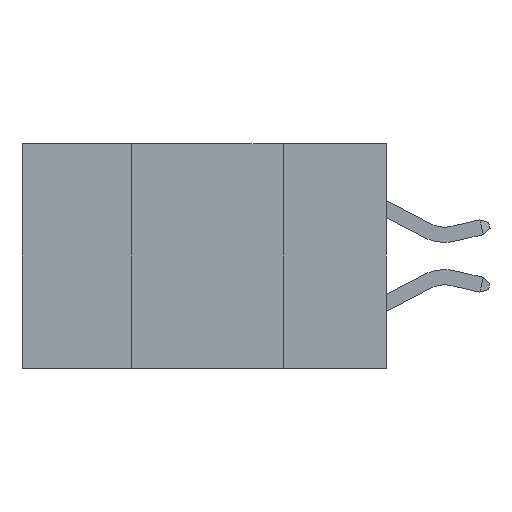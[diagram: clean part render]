
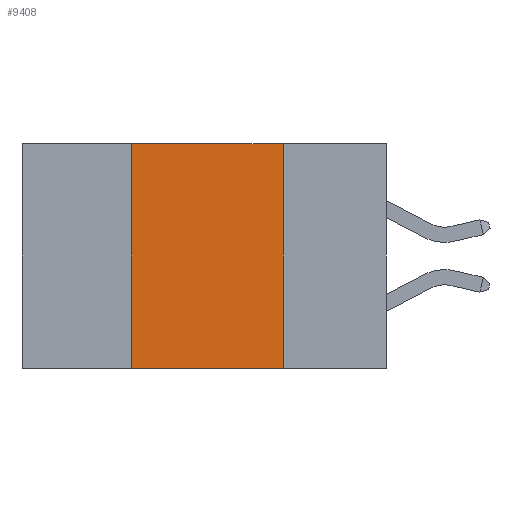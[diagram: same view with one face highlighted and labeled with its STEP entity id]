
A CAD part, left-side view. The second image highlights one B-rep face of the part: STEP entity #9408.
In plain terms, the highlighted planar face has unit normal (-1, 0, 0).
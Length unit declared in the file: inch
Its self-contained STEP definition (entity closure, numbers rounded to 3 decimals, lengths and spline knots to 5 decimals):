
#783 = EDGE_LOOP ( 'NONE', ( #13492, #8990, #10091, #8202 ) ) ;
#1760 = CARTESIAN_POINT ( 'NONE',  ( 0., 0.42, 0. ) ) ;
#1789 = EDGE_CURVE ( 'NONE', #5632, #4419, #1995, .T. ) ;
#1995 = LINE ( 'NONE', #13138, #7855 ) ;
#2279 = VERTEX_POINT ( 'NONE', #12585 ) ;
#2304 = CARTESIAN_POINT ( 'NONE',  ( 0., 0.6, 0. ) ) ;
#2442 = VERTEX_POINT ( 'NONE', #1760 ) ;
#3377 = LINE ( 'NONE', #14662, #12064 ) ;
#4105 = CARTESIAN_POINT ( 'NONE',  ( 0., 0.17, 0. ) ) ;
#4419 = VERTEX_POINT ( 'NONE', #9597 ) ;
#4425 = VECTOR ( 'NONE', #14667, 39.37008 ) ;
#5632 = VERTEX_POINT ( 'NONE', #7963 ) ;
#5768 = EDGE_CURVE ( 'NONE', #2442, #2279, #3377, .T. ) ;
#5909 = FACE_OUTER_BOUND ( 'NONE', #783, .T. ) ;
#7028 = PLANE ( 'NONE',  #13494 ) ;
#7406 = EDGE_CURVE ( 'NONE', #5632, #2442, #13409, .T. ) ;
#7855 = VECTOR ( 'NONE', #13776, 39.37008 ) ;
#7963 = CARTESIAN_POINT ( 'NONE',  ( 0., 0.42, -0.37 ) ) ;
#8176 = DIRECTION ( 'NONE',  ( 0., 0., -1. ) ) ;
#8202 = ORIENTED_EDGE ( 'NONE', *, *, #1789, .T. ) ;
#8990 = ORIENTED_EDGE ( 'NONE', *, *, #5768, .F. ) ;
#9077 = VECTOR ( 'NONE', #13130, 39.37008 ) ;
#9169 = CARTESIAN_POINT ( 'NONE',  ( 0., 0.42, 0. ) ) ;
#9408 = ADVANCED_FACE ( 'NONE', ( #5909 ), #7028, .F. ) ;
#9597 = CARTESIAN_POINT ( 'NONE',  ( 0., 0.17, -0.37 ) ) ;
#9721 = LINE ( 'NONE', #4105, #9077 ) ;
#10091 = ORIENTED_EDGE ( 'NONE', *, *, #7406, .F. ) ;
#10841 = EDGE_CURVE ( 'NONE', #2279, #4419, #9721, .T. ) ;
#12064 = VECTOR ( 'NONE', #14711, 39.37008 ) ;
#12585 = CARTESIAN_POINT ( 'NONE',  ( 0., 0.17, 0. ) ) ;
#13130 = DIRECTION ( 'NONE',  ( 0., 0., -1. ) ) ;
#13138 = CARTESIAN_POINT ( 'NONE',  ( 0., 0.6, -0.37 ) ) ;
#13409 = LINE ( 'NONE', #9169, #4425 ) ;
#13492 = ORIENTED_EDGE ( 'NONE', *, *, #10841, .F. ) ;
#13494 = AXIS2_PLACEMENT_3D ( 'NONE', #2304, #14800, #8176 ) ;
#13776 = DIRECTION ( 'NONE',  ( 0., -1., 0. ) ) ;
#14662 = CARTESIAN_POINT ( 'NONE',  ( 0., 0.6, 0. ) ) ;
#14667 = DIRECTION ( 'NONE',  ( 0., 0., 1. ) ) ;
#14711 = DIRECTION ( 'NONE',  ( 0., -1., 0. ) ) ;
#14800 = DIRECTION ( 'NONE',  ( 1., 0., 0. ) ) ;
